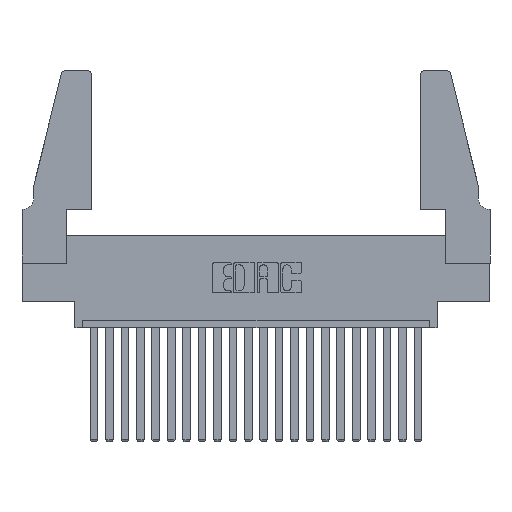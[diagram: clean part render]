
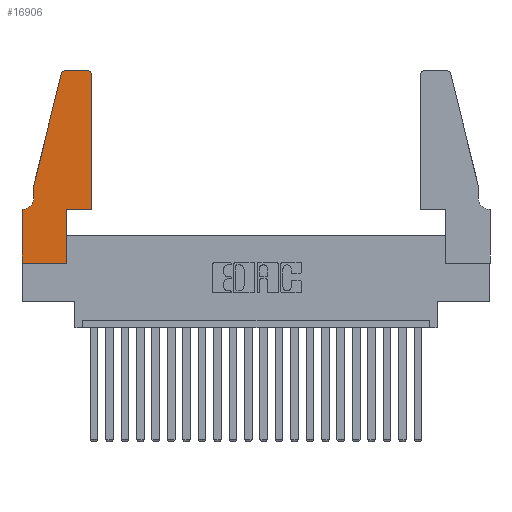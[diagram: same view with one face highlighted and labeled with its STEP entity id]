
A CAD part, top view. The second image highlights one B-rep face of the part: STEP entity #16906.
In plain terms, the highlighted planar face has unit normal (0, 0, 1).
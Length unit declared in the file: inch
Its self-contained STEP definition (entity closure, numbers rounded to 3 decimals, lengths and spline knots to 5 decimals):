
#143 = LINE ( 'NONE', #19009, #21294 ) ;
#978 = CARTESIAN_POINT ( 'NONE',  ( 0., 0.35, 0.37 ) ) ;
#1004 = VECTOR ( 'NONE', #1864, 39.37008 ) ;
#1060 = AXIS2_PLACEMENT_3D ( 'NONE', #978, #7310, #15588 ) ;
#1252 = AXIS2_PLACEMENT_3D ( 'NONE', #13822, #13591, #3981 ) ;
#1525 = EDGE_CURVE ( 'NONE', #18281, #15456, #1713, .T. ) ;
#1583 = DIRECTION ( 'NONE',  ( 0., 0., -1. ) ) ;
#1713 = CIRCLE ( 'NONE', #1252, 0.03 ) ;
#1864 = DIRECTION ( 'NONE',  ( 0., 1., 0. ) ) ;
#1900 = EDGE_CURVE ( 'NONE', #8812, #6546, #16408, .T. ) ;
#2415 = EDGE_CURVE ( 'NONE', #4172, #8812, #16411, .T. ) ;
#2550 = VERTEX_POINT ( 'NONE', #15295 ) ;
#2738 = CARTESIAN_POINT ( 'NONE',  ( 0.2605, 1.25, 0.37 ) ) ;
#2757 = ORIENTED_EDGE ( 'NONE', *, *, #6483, .T. ) ;
#2826 = ORIENTED_EDGE ( 'NONE', *, *, #18611, .T. ) ;
#3207 = DIRECTION ( 'NONE',  ( 0., 0., 1. ) ) ;
#3214 = VECTOR ( 'NONE', #13890, 39.37008 ) ;
#3275 = EDGE_CURVE ( 'NONE', #19720, #18281, #5219, .T. ) ;
#3981 = DIRECTION ( 'NONE',  ( 1., 0., 0. ) ) ;
#4172 = VERTEX_POINT ( 'NONE', #20999 ) ;
#4210 = FACE_OUTER_BOUND ( 'NONE', #11561, .T. ) ;
#4232 = EDGE_CURVE ( 'NONE', #2550, #11263, #14760, .T. ) ;
#4448 = CIRCLE ( 'NONE', #15433, 0.07 ) ;
#4864 = DIRECTION ( 'NONE',  ( 1., 0., 0. ) ) ;
#4924 = ORIENTED_EDGE ( 'NONE', *, *, #1525, .T. ) ;
#4984 = DIRECTION ( 'NONE',  ( -1., 0., 0. ) ) ;
#5219 = LINE ( 'NONE', #12380, #13240 ) ;
#5236 = CARTESIAN_POINT ( 'NONE',  ( 0.0755, 0.5, 0.37 ) ) ;
#5483 = CARTESIAN_POINT ( 'NONE',  ( 0., 0., 0.37 ) ) ;
#5798 = VECTOR ( 'NONE', #17224, 39.37008 ) ;
#5897 = CIRCLE ( 'NONE', #20456, 0.03 ) ;
#6483 = EDGE_CURVE ( 'NONE', #8053, #14073, #14891, .T. ) ;
#6546 = VERTEX_POINT ( 'NONE', #8654 ) ;
#6781 = DIRECTION ( 'NONE',  ( -0.239, -0.971, 0. ) ) ;
#7310 = DIRECTION ( 'NONE',  ( 0., 0., 1. ) ) ;
#7391 = DIRECTION ( 'NONE',  ( -1., 0., 0. ) ) ;
#7844 = CARTESIAN_POINT ( 'NONE',  ( 0.284, 1.25, 0.37 ) ) ;
#8053 = VERTEX_POINT ( 'NONE', #11599 ) ;
#8095 = ORIENTED_EDGE ( 'NONE', *, *, #16280, .T. ) ;
#8172 = CARTESIAN_POINT ( 'NONE',  ( 0.4505, 0.35, 0.37 ) ) ;
#8318 = EDGE_CURVE ( 'NONE', #16249, #4172, #4448, .T. ) ;
#8629 = ORIENTED_EDGE ( 'NONE', *, *, #21225, .T. ) ;
#8654 = CARTESIAN_POINT ( 'NONE',  ( 0., 0., 0.37 ) ) ;
#8812 = VERTEX_POINT ( 'NONE', #18967 ) ;
#9258 = CARTESIAN_POINT ( 'NONE',  ( 0.284, 1.22, 0.37 ) ) ;
#10263 = CARTESIAN_POINT ( 'NONE',  ( 0.2865, 0.35, 0.37 ) ) ;
#10738 = DIRECTION ( 'NONE',  ( 0., -1., 0. ) ) ;
#10896 = CARTESIAN_POINT ( 'NONE',  ( 0.0755, 0.35, 0.37 ) ) ;
#11263 = VERTEX_POINT ( 'NONE', #5236 ) ;
#11561 = EDGE_LOOP ( 'NONE', ( #19696, #8629, #20264, #8095, #13647, #19666, #14447, #19976, #2757, #2826, #19086, #4924 ) ) ;
#11599 = CARTESIAN_POINT ( 'NONE',  ( 0.2865, 0., 0.37 ) ) ;
#11647 = CARTESIAN_POINT ( 'NONE',  ( 0.0055, 0.42, 0.37 ) ) ;
#12272 = CARTESIAN_POINT ( 'NONE',  ( 0.0755, 0.42, 0.37 ) ) ;
#12380 = CARTESIAN_POINT ( 'NONE',  ( 0.4505, 0.35, 0.37 ) ) ;
#12679 = LINE ( 'NONE', #2738, #13163 ) ;
#13063 = CARTESIAN_POINT ( 'NONE',  ( 0.4505, 0.35, 0.37 ) ) ;
#13163 = VECTOR ( 'NONE', #7391, 39.37008 ) ;
#13240 = VECTOR ( 'NONE', #15504, 39.37008 ) ;
#13591 = DIRECTION ( 'NONE',  ( 0., 0., 1. ) ) ;
#13647 = ORIENTED_EDGE ( 'NONE', *, *, #8318, .T. ) ;
#13822 = CARTESIAN_POINT ( 'NONE',  ( 0.4205, 1.22, 0.37 ) ) ;
#13890 = DIRECTION ( 'NONE',  ( -1., 0., 0. ) ) ;
#13931 = PLANE ( 'NONE',  #1060 ) ;
#14073 = VERTEX_POINT ( 'NONE', #16510 ) ;
#14447 = ORIENTED_EDGE ( 'NONE', *, *, #1900, .T. ) ;
#14760 = LINE ( 'NONE', #18463, #15294 ) ;
#14891 = LINE ( 'NONE', #10263, #1004 ) ;
#14979 = CARTESIAN_POINT ( 'NONE',  ( 0.4205, 1.25, 0.37 ) ) ;
#15294 = VECTOR ( 'NONE', #6781, 39.37008 ) ;
#15295 = CARTESIAN_POINT ( 'NONE',  ( 0.25487, 1.22718, 0.37 ) ) ;
#15337 = LINE ( 'NONE', #8172, #20268 ) ;
#15433 = AXIS2_PLACEMENT_3D ( 'NONE', #11647, #1583, #4984 ) ;
#15456 = VERTEX_POINT ( 'NONE', #14979 ) ;
#15504 = DIRECTION ( 'NONE',  ( 0., 1., 0. ) ) ;
#15577 = EDGE_CURVE ( 'NONE', #6546, #8053, #17984, .T. ) ;
#15588 = DIRECTION ( 'NONE',  ( 1., 0., 0. ) ) ;
#15901 = CARTESIAN_POINT ( 'NONE',  ( 0.4505, 1.22, 0.37 ) ) ;
#16249 = VERTEX_POINT ( 'NONE', #12272 ) ;
#16280 = EDGE_CURVE ( 'NONE', #11263, #16249, #143, .T. ) ;
#16408 = LINE ( 'NONE', #17749, #20315 ) ;
#16411 = LINE ( 'NONE', #10896, #3214 ) ;
#16510 = CARTESIAN_POINT ( 'NONE',  ( 0.2865, 0.35, 0.37 ) ) ;
#16906 = ADVANCED_FACE ( 'NONE', ( #4210 ), #13931, .T. ) ;
#17224 = DIRECTION ( 'NONE',  ( 1., 0., 0. ) ) ;
#17749 = CARTESIAN_POINT ( 'NONE',  ( 0., 0., 0.37 ) ) ;
#17984 = LINE ( 'NONE', #5483, #5798 ) ;
#18281 = VERTEX_POINT ( 'NONE', #15901 ) ;
#18463 = CARTESIAN_POINT ( 'NONE',  ( 0.0755, 0.5, 0.37 ) ) ;
#18611 = EDGE_CURVE ( 'NONE', #14073, #19720, #15337, .T. ) ;
#18967 = CARTESIAN_POINT ( 'NONE',  ( 0., 0.35, 0.37 ) ) ;
#19009 = CARTESIAN_POINT ( 'NONE',  ( 0.0755, 0.5, 0.37 ) ) ;
#19086 = ORIENTED_EDGE ( 'NONE', *, *, #3275, .T. ) ;
#19637 = VERTEX_POINT ( 'NONE', #7844 ) ;
#19666 = ORIENTED_EDGE ( 'NONE', *, *, #2415, .T. ) ;
#19696 = ORIENTED_EDGE ( 'NONE', *, *, #20688, .T. ) ;
#19720 = VERTEX_POINT ( 'NONE', #13063 ) ;
#19798 = DIRECTION ( 'NONE',  ( 1., 0., 0. ) ) ;
#19976 = ORIENTED_EDGE ( 'NONE', *, *, #15577, .T. ) ;
#20264 = ORIENTED_EDGE ( 'NONE', *, *, #4232, .T. ) ;
#20268 = VECTOR ( 'NONE', #19798, 39.37008 ) ;
#20315 = VECTOR ( 'NONE', #21060, 39.37008 ) ;
#20456 = AXIS2_PLACEMENT_3D ( 'NONE', #9258, #3207, #4864 ) ;
#20688 = EDGE_CURVE ( 'NONE', #15456, #19637, #12679, .T. ) ;
#20999 = CARTESIAN_POINT ( 'NONE',  ( 0.0055, 0.35, 0.37 ) ) ;
#21060 = DIRECTION ( 'NONE',  ( 0., -1., 0. ) ) ;
#21225 = EDGE_CURVE ( 'NONE', #19637, #2550, #5897, .T. ) ;
#21294 = VECTOR ( 'NONE', #10738, 39.37008 ) ;
